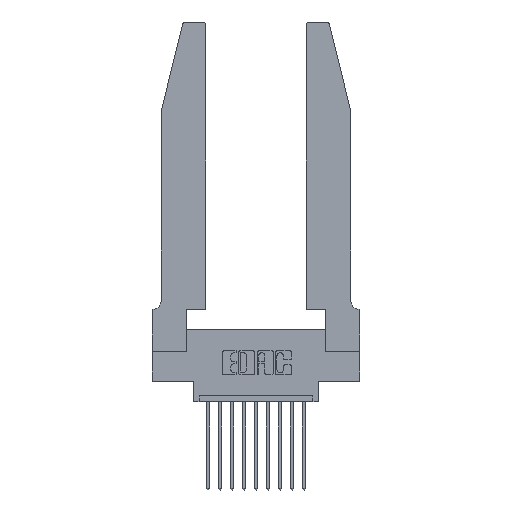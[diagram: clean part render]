
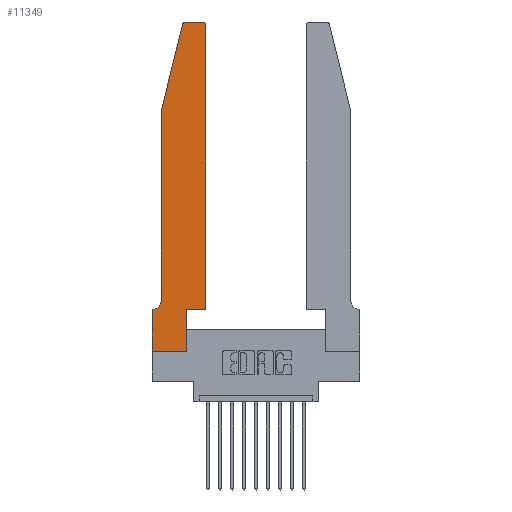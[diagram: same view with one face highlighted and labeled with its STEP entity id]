
A CAD part, top view. The second image highlights one B-rep face of the part: STEP entity #11349.
In plain terms, the highlighted planar face has unit normal (0, 0, 1).
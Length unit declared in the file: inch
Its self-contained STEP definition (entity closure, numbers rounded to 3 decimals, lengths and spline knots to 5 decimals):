
#30 = VERTEX_POINT ( 'NONE', #10325 ) ;
#177 = VECTOR ( 'NONE', #5354, 39.37008 ) ;
#271 = DIRECTION ( 'NONE',  ( 1., 0., 0. ) ) ;
#599 = DIRECTION ( 'NONE',  ( 1., 0., 0. ) ) ;
#721 = AXIS2_PLACEMENT_3D ( 'NONE', #8916, #5263, #5318 ) ;
#753 = CARTESIAN_POINT ( 'NONE',  ( 0., 0.35, 0.37 ) ) ;
#814 = CARTESIAN_POINT ( 'NONE',  ( 0., 0., 0.37 ) ) ;
#1007 = EDGE_CURVE ( 'NONE', #7255, #15962, #7221, .T. ) ;
#1287 = CARTESIAN_POINT ( 'NONE',  ( 0.284, 2.72, 0.37 ) ) ;
#1333 = LINE ( 'NONE', #6162, #13797 ) ;
#1570 = LINE ( 'NONE', #4677, #6092 ) ;
#1744 = VERTEX_POINT ( 'NONE', #5548 ) ;
#1814 = VERTEX_POINT ( 'NONE', #753 ) ;
#1871 = VERTEX_POINT ( 'NONE', #8396 ) ;
#1933 = ORIENTED_EDGE ( 'NONE', *, *, #1007, .T. ) ;
#2267 = DIRECTION ( 'NONE',  ( 0., -1., 0. ) ) ;
#2392 = ORIENTED_EDGE ( 'NONE', *, *, #3807, .T. ) ;
#2397 = AXIS2_PLACEMENT_3D ( 'NONE', #1287, #11237, #13585 ) ;
#2534 = DIRECTION ( 'NONE',  ( 1., 0., 0. ) ) ;
#2538 = VECTOR ( 'NONE', #6701, 39.37008 ) ;
#2687 = VERTEX_POINT ( 'NONE', #814 ) ;
#2860 = DIRECTION ( 'NONE',  ( 0., 0., 1. ) ) ;
#2905 = DIRECTION ( 'NONE',  ( -1., 0., 0. ) ) ;
#2925 = VECTOR ( 'NONE', #599, 39.37008 ) ;
#2981 = ORIENTED_EDGE ( 'NONE', *, *, #13203, .T. ) ;
#3033 = ORIENTED_EDGE ( 'NONE', *, *, #13125, .T. ) ;
#3184 = VECTOR ( 'NONE', #12986, 39.37008 ) ;
#3367 = ORIENTED_EDGE ( 'NONE', *, *, #14406, .T. ) ;
#3662 = ORIENTED_EDGE ( 'NONE', *, *, #7040, .T. ) ;
#3681 = CARTESIAN_POINT ( 'NONE',  ( 0.0755, 2., 0.37 ) ) ;
#3807 = EDGE_CURVE ( 'NONE', #13917, #13189, #5804, .T. ) ;
#3819 = ORIENTED_EDGE ( 'NONE', *, *, #12301, .T. ) ;
#4260 = CARTESIAN_POINT ( 'NONE',  ( 0.2865, 0.35, 0.37 ) ) ;
#4677 = CARTESIAN_POINT ( 'NONE',  ( 0., 0., 0.37 ) ) ;
#4702 = CARTESIAN_POINT ( 'NONE',  ( 0.2865, 0.35, 0.37 ) ) ;
#5181 = ORIENTED_EDGE ( 'NONE', *, *, #12988, .T. ) ;
#5263 = DIRECTION ( 'NONE',  ( 0., 0., 1. ) ) ;
#5318 = DIRECTION ( 'NONE',  ( 1., 0., 0. ) ) ;
#5354 = DIRECTION ( 'NONE',  ( 0., 1., 0. ) ) ;
#5383 = CARTESIAN_POINT ( 'NONE',  ( 0.4205, 2.72, 0.37 ) ) ;
#5548 = CARTESIAN_POINT ( 'NONE',  ( 0.284, 2.75, 0.37 ) ) ;
#5647 = CIRCLE ( 'NONE', #2397, 0.03 ) ;
#5737 = VERTEX_POINT ( 'NONE', #15829 ) ;
#5750 = CARTESIAN_POINT ( 'NONE',  ( 0.2865, 0., 0.37 ) ) ;
#5804 = LINE ( 'NONE', #12843, #12975 ) ;
#5874 = ORIENTED_EDGE ( 'NONE', *, *, #14077, .T. ) ;
#6019 = EDGE_CURVE ( 'NONE', #15962, #5737, #13455, .T. ) ;
#6092 = VECTOR ( 'NONE', #2267, 39.37008 ) ;
#6162 = CARTESIAN_POINT ( 'NONE',  ( 0.2605, 2.75, 0.37 ) ) ;
#6401 = CARTESIAN_POINT ( 'NONE',  ( 0.0755, 0.42, 0.37 ) ) ;
#6424 = VERTEX_POINT ( 'NONE', #10797 ) ;
#6701 = DIRECTION ( 'NONE',  ( 0., 1., 0. ) ) ;
#7040 = EDGE_CURVE ( 'NONE', #30, #7467, #13226, .T. ) ;
#7165 = EDGE_CURVE ( 'NONE', #2687, #7255, #14945, .T. ) ;
#7221 = LINE ( 'NONE', #4260, #177 ) ;
#7255 = VERTEX_POINT ( 'NONE', #5750 ) ;
#7367 = AXIS2_PLACEMENT_3D ( 'NONE', #5383, #2860, #271 ) ;
#7448 = DIRECTION ( 'NONE',  ( -1., 0., 0. ) ) ;
#7467 = VERTEX_POINT ( 'NONE', #8676 ) ;
#7643 = DIRECTION ( 'NONE',  ( 0., 0., -1. ) ) ;
#8396 = CARTESIAN_POINT ( 'NONE',  ( 0.0055, 0.35, 0.37 ) ) ;
#8676 = CARTESIAN_POINT ( 'NONE',  ( 0.4205, 2.75, 0.37 ) ) ;
#8801 = LINE ( 'NONE', #14299, #3184 ) ;
#8916 = CARTESIAN_POINT ( 'NONE',  ( 0., 0.35, 0.37 ) ) ;
#9201 = FACE_OUTER_BOUND ( 'NONE', #9415, .T. ) ;
#9415 = EDGE_LOOP ( 'NONE', ( #5874, #11398, #3033, #2392, #2981, #3819, #5181, #13513, #1933, #12129, #3367, #3662 ) ) ;
#9747 = CARTESIAN_POINT ( 'NONE',  ( 0.4505, 0.35, 0.37 ) ) ;
#10058 = DIRECTION ( 'NONE',  ( -0.239, -0.971, 0. ) ) ;
#10182 = CARTESIAN_POINT ( 'NONE',  ( 0.4505, 0.35, 0.37 ) ) ;
#10325 = CARTESIAN_POINT ( 'NONE',  ( 0.4505, 2.72, 0.37 ) ) ;
#10566 = DIRECTION ( 'NONE',  ( 0., -1., 0. ) ) ;
#10797 = CARTESIAN_POINT ( 'NONE',  ( 0.25487, 2.72718, 0.37 ) ) ;
#10890 = AXIS2_PLACEMENT_3D ( 'NONE', #12828, #7643, #2905 ) ;
#11101 = VECTOR ( 'NONE', #10058, 39.37008 ) ;
#11237 = DIRECTION ( 'NONE',  ( 0., 0., 1. ) ) ;
#11349 = ADVANCED_FACE ( 'NONE', ( #9201 ), #12730, .T. ) ;
#11398 = ORIENTED_EDGE ( 'NONE', *, *, #15536, .T. ) ;
#11489 = CIRCLE ( 'NONE', #10890, 0.07 ) ;
#11786 = CARTESIAN_POINT ( 'NONE',  ( 0.0755, 2., 0.37 ) ) ;
#12129 = ORIENTED_EDGE ( 'NONE', *, *, #6019, .T. ) ;
#12301 = EDGE_CURVE ( 'NONE', #1871, #1814, #8801, .T. ) ;
#12422 = LINE ( 'NONE', #10182, #2538 ) ;
#12730 = PLANE ( 'NONE',  #721 ) ;
#12828 = CARTESIAN_POINT ( 'NONE',  ( 0.0055, 0.42, 0.37 ) ) ;
#12843 = CARTESIAN_POINT ( 'NONE',  ( 0.0755, 2., 0.37 ) ) ;
#12975 = VECTOR ( 'NONE', #10566, 39.37008 ) ;
#12986 = DIRECTION ( 'NONE',  ( -1., 0., 0. ) ) ;
#12988 = EDGE_CURVE ( 'NONE', #1814, #2687, #1570, .T. ) ;
#13125 = EDGE_CURVE ( 'NONE', #6424, #13917, #15172, .T. ) ;
#13189 = VERTEX_POINT ( 'NONE', #6401 ) ;
#13203 = EDGE_CURVE ( 'NONE', #13189, #1871, #11489, .T. ) ;
#13226 = CIRCLE ( 'NONE', #7367, 0.03 ) ;
#13455 = LINE ( 'NONE', #9747, #15968 ) ;
#13513 = ORIENTED_EDGE ( 'NONE', *, *, #7165, .T. ) ;
#13585 = DIRECTION ( 'NONE',  ( 1., 0., 0. ) ) ;
#13797 = VECTOR ( 'NONE', #7448, 39.37008 ) ;
#13917 = VERTEX_POINT ( 'NONE', #11786 ) ;
#14077 = EDGE_CURVE ( 'NONE', #7467, #1744, #1333, .T. ) ;
#14299 = CARTESIAN_POINT ( 'NONE',  ( 0.0755, 0.35, 0.37 ) ) ;
#14406 = EDGE_CURVE ( 'NONE', #5737, #30, #12422, .T. ) ;
#14945 = LINE ( 'NONE', #15560, #2925 ) ;
#15172 = LINE ( 'NONE', #3681, #11101 ) ;
#15536 = EDGE_CURVE ( 'NONE', #1744, #6424, #5647, .T. ) ;
#15560 = CARTESIAN_POINT ( 'NONE',  ( 0., 0., 0.37 ) ) ;
#15829 = CARTESIAN_POINT ( 'NONE',  ( 0.4505, 0.35, 0.37 ) ) ;
#15962 = VERTEX_POINT ( 'NONE', #4702 ) ;
#15968 = VECTOR ( 'NONE', #2534, 39.37008 ) ;
